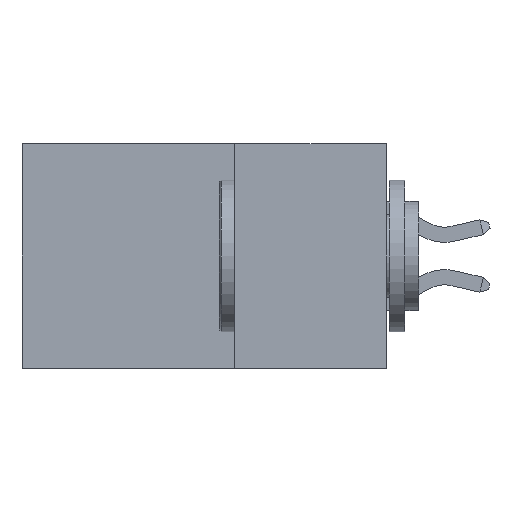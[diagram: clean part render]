
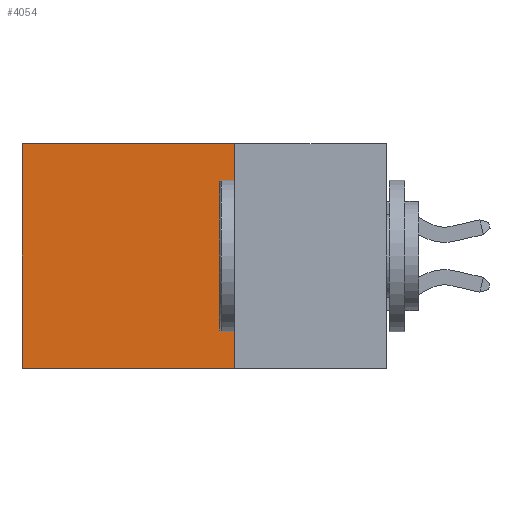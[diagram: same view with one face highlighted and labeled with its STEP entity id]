
A CAD part, left-side view. The second image highlights one B-rep face of the part: STEP entity #4054.
In plain terms, the highlighted planar face has unit normal (-1, 0, 0).
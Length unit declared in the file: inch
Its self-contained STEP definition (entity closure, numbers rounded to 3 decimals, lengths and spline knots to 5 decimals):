
#416 = CARTESIAN_POINT ( 'NONE',  ( 0.298, 0.6, -0.37 ) ) ;
#462 = CARTESIAN_POINT ( 'NONE',  ( 0.298, 0.6, 0. ) ) ;
#484 = LINE ( 'NONE', #462, #9348 ) ;
#858 = CARTESIAN_POINT ( 'NONE',  ( 0.298, 0.6, 0. ) ) ;
#1218 = DIRECTION ( 'NONE',  ( 0., 0., -1. ) ) ;
#1366 = ORIENTED_EDGE ( 'NONE', *, *, #1967, .F. ) ;
#1718 = DIRECTION ( 'NONE',  ( 0., 1., 0. ) ) ;
#1742 = ORIENTED_EDGE ( 'NONE', *, *, #7978, .F. ) ;
#1803 = EDGE_CURVE ( 'NONE', #10204, #5770, #9316, .T. ) ;
#1967 = EDGE_CURVE ( 'NONE', #10167, #3439, #8322, .T. ) ;
#2918 = CARTESIAN_POINT ( 'NONE',  ( 0.298, 0.25, -0.37 ) ) ;
#3350 = CARTESIAN_POINT ( 'NONE',  ( 0.298, 0.25, 0. ) ) ;
#3439 = VERTEX_POINT ( 'NONE', #416 ) ;
#3671 = DIRECTION ( 'NONE',  ( 0., 0., -1. ) ) ;
#4054 = ADVANCED_FACE ( 'NONE', ( #8022 ), #4932, .F. ) ;
#4490 = CARTESIAN_POINT ( 'NONE',  ( 0.298, 0.25, 0. ) ) ;
#4750 = CARTESIAN_POINT ( 'NONE',  ( 0.298, 0.25, -0.37 ) ) ;
#4932 = PLANE ( 'NONE',  #9116 ) ;
#5132 = VECTOR ( 'NONE', #1718, 39.37008 ) ;
#5673 = CARTESIAN_POINT ( 'NONE',  ( 0.298, 0.25, 0. ) ) ;
#5770 = VERTEX_POINT ( 'NONE', #858 ) ;
#6107 = EDGE_CURVE ( 'NONE', #5770, #3439, #484, .T. ) ;
#6446 = LINE ( 'NONE', #7581, #7049 ) ;
#6608 = VECTOR ( 'NONE', #8028, 39.37008 ) ;
#7049 = VECTOR ( 'NONE', #3671, 39.37008 ) ;
#7243 = ORIENTED_EDGE ( 'NONE', *, *, #6107, .T. ) ;
#7581 = CARTESIAN_POINT ( 'NONE',  ( 0.298, 0.25, 0. ) ) ;
#7978 = EDGE_CURVE ( 'NONE', #10204, #10167, #6446, .T. ) ;
#8022 = FACE_OUTER_BOUND ( 'NONE', #8105, .T. ) ;
#8028 = DIRECTION ( 'NONE',  ( 0., 1., 0. ) ) ;
#8105 = EDGE_LOOP ( 'NONE', ( #7243, #1366, #1742, #9990 ) ) ;
#8322 = LINE ( 'NONE', #4750, #5132 ) ;
#9116 = AXIS2_PLACEMENT_3D ( 'NONE', #3350, #9565, #9671 ) ;
#9316 = LINE ( 'NONE', #5673, #6608 ) ;
#9348 = VECTOR ( 'NONE', #1218, 39.37008 ) ;
#9565 = DIRECTION ( 'NONE',  ( 1., 0., 0. ) ) ;
#9671 = DIRECTION ( 'NONE',  ( 0., 0., -1. ) ) ;
#9990 = ORIENTED_EDGE ( 'NONE', *, *, #1803, .T. ) ;
#10167 = VERTEX_POINT ( 'NONE', #2918 ) ;
#10204 = VERTEX_POINT ( 'NONE', #4490 ) ;
